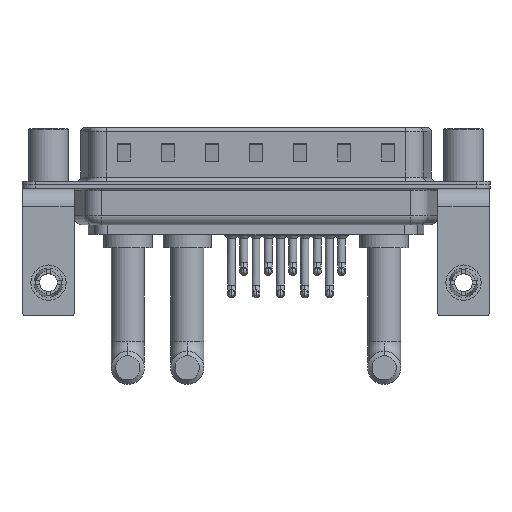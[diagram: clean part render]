
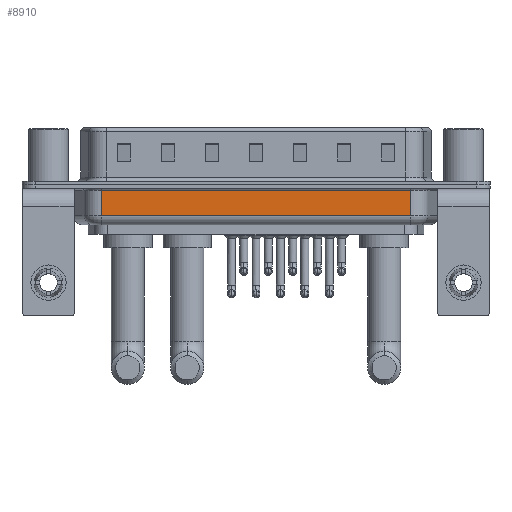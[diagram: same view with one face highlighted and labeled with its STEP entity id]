
A CAD part, front view. The second image highlights one B-rep face of the part: STEP entity #8910.
In plain terms, the highlighted planar face has unit normal (0, -1, 0).
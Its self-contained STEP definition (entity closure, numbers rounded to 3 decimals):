
#940 = CARTESIAN_POINT ( 'NONE',  ( 41.044, -5.35, -0.65 ) ) ;
#1643 = PLANE ( 'NONE',  #22162 ) ;
#1929 = CARTESIAN_POINT ( 'NONE',  ( 6.006, -5.35, -4.5 ) ) ;
#2012 = VECTOR ( 'NONE', #8375, 1000. ) ;
#2638 = ORIENTED_EDGE ( 'NONE', *, *, #11111, .T. ) ;
#4027 = CARTESIAN_POINT ( 'NONE',  ( 6.006, -5.35, -0.65 ) ) ;
#5138 = DIRECTION ( 'NONE',  ( 1., 0., 0. ) ) ;
#5284 = LINE ( 'NONE', #27238, #16829 ) ;
#5557 = CARTESIAN_POINT ( 'NONE',  ( 6.006, -5.35, -3.5 ) ) ;
#5598 = EDGE_CURVE ( 'NONE', #20249, #15986, #18318, .T. ) ;
#6062 = DIRECTION ( 'NONE',  ( -1., 0., 0. ) ) ;
#6245 = DIRECTION ( 'NONE',  ( 0., 0., 1. ) ) ;
#6529 = LINE ( 'NONE', #1929, #2012 ) ;
#7991 = VERTEX_POINT ( 'NONE', #18276 ) ;
#8375 = DIRECTION ( 'NONE',  ( 0., 0., 1. ) ) ;
#8609 = EDGE_LOOP ( 'NONE', ( #13033, #2638, #19414, #13815 ) ) ;
#8910 = ADVANCED_FACE ( 'NONE', ( #16922 ), #1643, .F. ) ;
#9206 = CARTESIAN_POINT ( 'NONE',  ( 41.044, -5.35, -4.5 ) ) ;
#9510 = LINE ( 'NONE', #5557, #16833 ) ;
#10406 = VERTEX_POINT ( 'NONE', #4027 ) ;
#10487 = EDGE_CURVE ( 'NONE', #7991, #10406, #6529, .T. ) ;
#11111 = EDGE_CURVE ( 'NONE', #7991, #20249, #9510, .T. ) ;
#12569 = EDGE_CURVE ( 'NONE', #15986, #10406, #5284, .T. ) ;
#13033 = ORIENTED_EDGE ( 'NONE', *, *, #10487, .F. ) ;
#13815 = ORIENTED_EDGE ( 'NONE', *, *, #12569, .T. ) ;
#15986 = VERTEX_POINT ( 'NONE', #940 ) ;
#16829 = VECTOR ( 'NONE', #6062, 1000. ) ;
#16833 = VECTOR ( 'NONE', #5138, 1000. ) ;
#16922 = FACE_OUTER_BOUND ( 'NONE', #8609, .T. ) ;
#18276 = CARTESIAN_POINT ( 'NONE',  ( 6.006, -5.35, -3.5 ) ) ;
#18318 = LINE ( 'NONE', #9206, #22387 ) ;
#19414 = ORIENTED_EDGE ( 'NONE', *, *, #5598, .T. ) ;
#20249 = VERTEX_POINT ( 'NONE', #22512 ) ;
#20275 = DIRECTION ( 'NONE',  ( 0., 0., 1. ) ) ;
#22162 = AXIS2_PLACEMENT_3D ( 'NONE', #23207, #25455, #6245 ) ;
#22387 = VECTOR ( 'NONE', #20275, 1000. ) ;
#22512 = CARTESIAN_POINT ( 'NONE',  ( 41.044, -5.35, -3.5 ) ) ;
#23207 = CARTESIAN_POINT ( 'NONE',  ( 6.006, -5.35, -4.5 ) ) ;
#25455 = DIRECTION ( 'NONE',  ( 0., 1., 0. ) ) ;
#27238 = CARTESIAN_POINT ( 'NONE',  ( 6.006, -5.35, -0.65 ) ) ;
